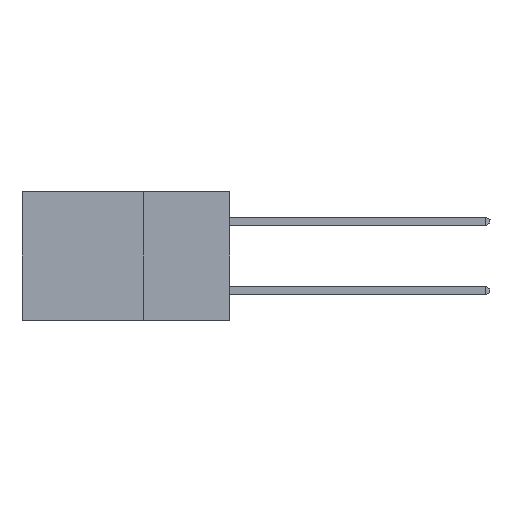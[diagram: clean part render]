
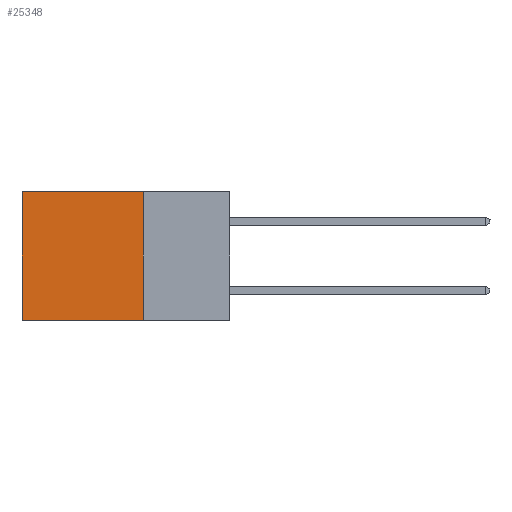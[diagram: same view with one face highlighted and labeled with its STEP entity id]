
A CAD part, left-side view. The second image highlights one B-rep face of the part: STEP entity #25348.
In plain terms, the highlighted planar face has unit normal (-1, 0, 0).
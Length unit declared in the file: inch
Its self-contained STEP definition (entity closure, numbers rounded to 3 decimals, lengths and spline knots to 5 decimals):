
#2833 = VERTEX_POINT ( 'NONE', #6576 ) ;
#3105 = VERTEX_POINT ( 'NONE', #23504 ) ;
#3259 = DIRECTION ( 'NONE',  ( 0., 0., -1. ) ) ;
#4272 = CARTESIAN_POINT ( 'NONE',  ( 0.298, 0.6, -0.37 ) ) ;
#4460 = DIRECTION ( 'NONE',  ( 0., 1., 0. ) ) ;
#5065 = LINE ( 'NONE', #25822, #30898 ) ;
#5929 = VERTEX_POINT ( 'NONE', #4272 ) ;
#5999 = CARTESIAN_POINT ( 'NONE',  ( 0.298, 0.25, 0. ) ) ;
#6576 = CARTESIAN_POINT ( 'NONE',  ( 0.298, 0.25, -0.37 ) ) ;
#7412 = EDGE_CURVE ( 'NONE', #21535, #3105, #27369, .T. ) ;
#8125 = LINE ( 'NONE', #17067, #27335 ) ;
#8577 = DIRECTION ( 'NONE',  ( 0., 1., 0. ) ) ;
#9294 = ORIENTED_EDGE ( 'NONE', *, *, #10709, .F. ) ;
#10709 = EDGE_CURVE ( 'NONE', #2833, #5929, #25369, .T. ) ;
#10948 = FACE_OUTER_BOUND ( 'NONE', #18108, .T. ) ;
#14112 = VECTOR ( 'NONE', #8577, 39.37008 ) ;
#14170 = DIRECTION ( 'NONE',  ( 1., 0., 0. ) ) ;
#16514 = ORIENTED_EDGE ( 'NONE', *, *, #32280, .T. ) ;
#17067 = CARTESIAN_POINT ( 'NONE',  ( 0.298, 0.6, 0. ) ) ;
#18108 = EDGE_LOOP ( 'NONE', ( #16514, #9294, #20704, #23100 ) ) ;
#19607 = DIRECTION ( 'NONE',  ( 0., 0., -1. ) ) ;
#19643 = CARTESIAN_POINT ( 'NONE',  ( 0.298, 0.25, -0.37 ) ) ;
#20704 = ORIENTED_EDGE ( 'NONE', *, *, #28248, .F. ) ;
#21535 = VERTEX_POINT ( 'NONE', #31271 ) ;
#23100 = ORIENTED_EDGE ( 'NONE', *, *, #7412, .T. ) ;
#23504 = CARTESIAN_POINT ( 'NONE',  ( 0.298, 0.6, 0. ) ) ;
#25348 = ADVANCED_FACE ( 'NONE', ( #10948 ), #29017, .F. ) ;
#25369 = LINE ( 'NONE', #19643, #26139 ) ;
#25822 = CARTESIAN_POINT ( 'NONE',  ( 0.298, 0.25, 0. ) ) ;
#26139 = VECTOR ( 'NONE', #4460, 39.37008 ) ;
#27335 = VECTOR ( 'NONE', #19607, 39.37008 ) ;
#27369 = LINE ( 'NONE', #5999, #14112 ) ;
#28248 = EDGE_CURVE ( 'NONE', #21535, #2833, #5065, .T. ) ;
#29017 = PLANE ( 'NONE',  #30283 ) ;
#30283 = AXIS2_PLACEMENT_3D ( 'NONE', #31433, #14170, #31545 ) ;
#30898 = VECTOR ( 'NONE', #3259, 39.37008 ) ;
#31271 = CARTESIAN_POINT ( 'NONE',  ( 0.298, 0.25, 0. ) ) ;
#31433 = CARTESIAN_POINT ( 'NONE',  ( 0.298, 0.25, 0. ) ) ;
#31545 = DIRECTION ( 'NONE',  ( 0., 0., -1. ) ) ;
#32280 = EDGE_CURVE ( 'NONE', #3105, #5929, #8125, .T. ) ;
